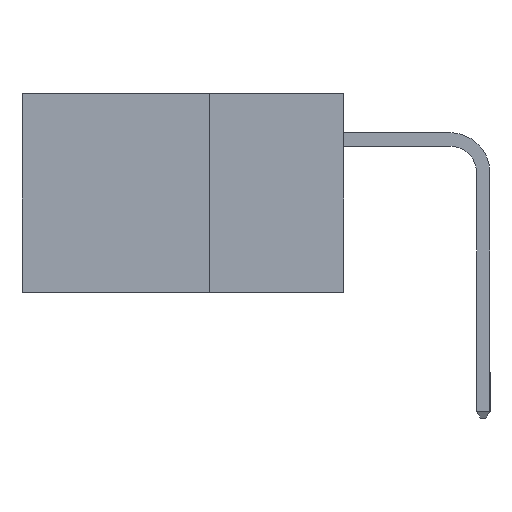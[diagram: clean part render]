
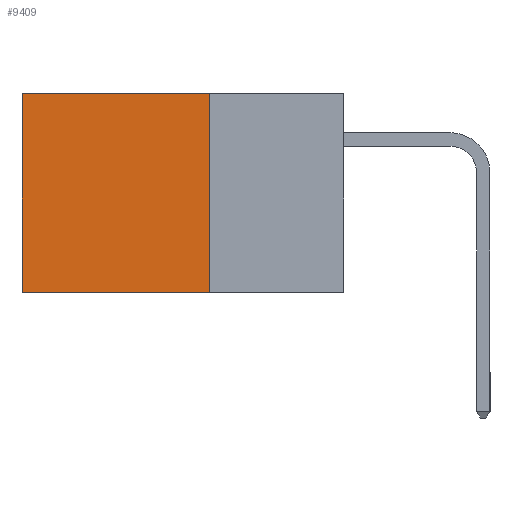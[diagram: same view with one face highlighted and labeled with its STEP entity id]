
A CAD part, left-side view. The second image highlights one B-rep face of the part: STEP entity #9409.
In plain terms, the highlighted planar face has unit normal (-1, 0, 0).
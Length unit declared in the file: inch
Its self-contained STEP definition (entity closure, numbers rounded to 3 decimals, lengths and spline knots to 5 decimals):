
#491 = EDGE_CURVE ( 'NONE', #2349, #10889, #9690, .T. ) ;
#1227 = DIRECTION ( 'NONE',  ( 0., 1., 0. ) ) ;
#2264 = AXIS2_PLACEMENT_3D ( 'NONE', #6275, #11684, #5315 ) ;
#2349 = VERTEX_POINT ( 'NONE', #6274 ) ;
#2434 = FACE_OUTER_BOUND ( 'NONE', #11563, .T. ) ;
#2918 = VERTEX_POINT ( 'NONE', #10142 ) ;
#3184 = LINE ( 'NONE', #6850, #10597 ) ;
#3569 = PLANE ( 'NONE',  #2264 ) ;
#3844 = EDGE_CURVE ( 'NONE', #2349, #3892, #3943, .T. ) ;
#3892 = VERTEX_POINT ( 'NONE', #4728 ) ;
#3943 = LINE ( 'NONE', #10219, #6576 ) ;
#4030 = ORIENTED_EDGE ( 'NONE', *, *, #4786, .T. ) ;
#4205 = LINE ( 'NONE', #8633, #5243 ) ;
#4728 = CARTESIAN_POINT ( 'NONE',  ( 0.2615, 0.6, 0. ) ) ;
#4786 = EDGE_CURVE ( 'NONE', #3892, #2918, #4205, .T. ) ;
#4844 = EDGE_CURVE ( 'NONE', #10889, #2918, #3184, .T. ) ;
#5243 = VECTOR ( 'NONE', #6729, 39.37008 ) ;
#5315 = DIRECTION ( 'NONE',  ( 0., 0., -1. ) ) ;
#5532 = ORIENTED_EDGE ( 'NONE', *, *, #4844, .F. ) ;
#6166 = DIRECTION ( 'NONE',  ( 0., 0., -1. ) ) ;
#6274 = CARTESIAN_POINT ( 'NONE',  ( 0.2615, 0.25, 0. ) ) ;
#6275 = CARTESIAN_POINT ( 'NONE',  ( 0.2615, 0.25, -0.37 ) ) ;
#6576 = VECTOR ( 'NONE', #1227, 39.37008 ) ;
#6729 = DIRECTION ( 'NONE',  ( 0., 0., -1. ) ) ;
#6850 = CARTESIAN_POINT ( 'NONE',  ( 0.2615, 0.25, -0.37 ) ) ;
#8633 = CARTESIAN_POINT ( 'NONE',  ( 0.2615, 0.6, -0.37 ) ) ;
#8676 = VECTOR ( 'NONE', #6166, 39.37008 ) ;
#8896 = CARTESIAN_POINT ( 'NONE',  ( 0.2615, 0.25, -0.37 ) ) ;
#9409 = ADVANCED_FACE ( 'NONE', ( #2434 ), #3569, .F. ) ;
#9690 = LINE ( 'NONE', #11525, #8676 ) ;
#10142 = CARTESIAN_POINT ( 'NONE',  ( 0.2615, 0.6, -0.37 ) ) ;
#10219 = CARTESIAN_POINT ( 'NONE',  ( 0.2615, 0.25, 0. ) ) ;
#10597 = VECTOR ( 'NONE', #10602, 39.37008 ) ;
#10602 = DIRECTION ( 'NONE',  ( 0., 1., 0. ) ) ;
#10889 = VERTEX_POINT ( 'NONE', #8896 ) ;
#11007 = ORIENTED_EDGE ( 'NONE', *, *, #3844, .T. ) ;
#11295 = ORIENTED_EDGE ( 'NONE', *, *, #491, .F. ) ;
#11525 = CARTESIAN_POINT ( 'NONE',  ( 0.2615, 0.25, -0.37 ) ) ;
#11563 = EDGE_LOOP ( 'NONE', ( #4030, #5532, #11295, #11007 ) ) ;
#11684 = DIRECTION ( 'NONE',  ( 1., 0., 0. ) ) ;
